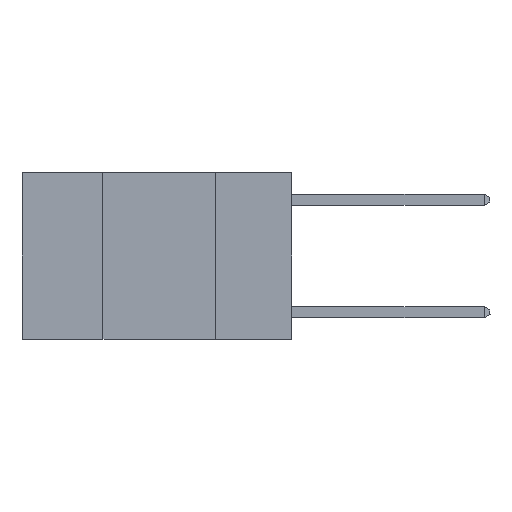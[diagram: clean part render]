
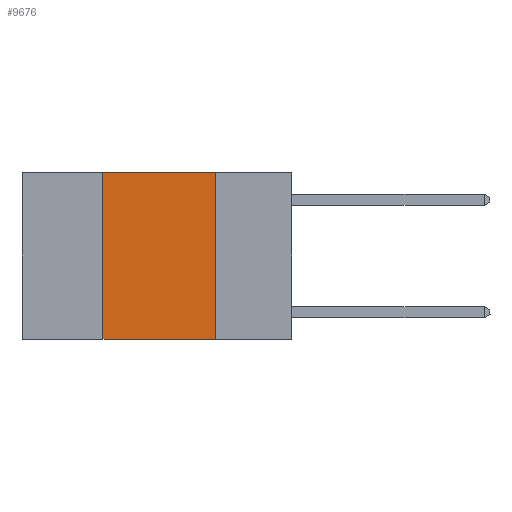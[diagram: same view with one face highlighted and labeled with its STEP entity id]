
A CAD part, left-side view. The second image highlights one B-rep face of the part: STEP entity #9676.
In plain terms, the highlighted planar face has unit normal (-1, 0, 0).
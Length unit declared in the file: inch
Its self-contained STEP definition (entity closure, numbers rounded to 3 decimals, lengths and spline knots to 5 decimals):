
#688 = DIRECTION ( 'NONE',  ( 0., 0., 1. ) ) ;
#775 = EDGE_CURVE ( 'NONE', #9578, #14769, #13753, .T. ) ;
#1675 = FACE_OUTER_BOUND ( 'NONE', #10880, .T. ) ;
#1906 = ORIENTED_EDGE ( 'NONE', *, *, #775, .F. ) ;
#2052 = CARTESIAN_POINT ( 'NONE',  ( 0., 0.17, -0.37 ) ) ;
#2343 = ORIENTED_EDGE ( 'NONE', *, *, #8108, .F. ) ;
#3382 = CARTESIAN_POINT ( 'NONE',  ( 0., 0.42, 0. ) ) ;
#4011 = DIRECTION ( 'NONE',  ( 0., 0., -1. ) ) ;
#4196 = DIRECTION ( 'NONE',  ( 0., 0., -1. ) ) ;
#4293 = VECTOR ( 'NONE', #688, 39.37008 ) ;
#4653 = VECTOR ( 'NONE', #15458, 39.37008 ) ;
#4660 = LINE ( 'NONE', #11481, #14763 ) ;
#4905 = CARTESIAN_POINT ( 'NONE',  ( 0., 0.6, -0.37 ) ) ;
#5914 = ORIENTED_EDGE ( 'NONE', *, *, #16284, .T. ) ;
#8107 = DIRECTION ( 'NONE',  ( 1., 0., 0. ) ) ;
#8108 = EDGE_CURVE ( 'NONE', #10949, #14846, #8243, .T. ) ;
#8243 = LINE ( 'NONE', #3382, #4293 ) ;
#8591 = LINE ( 'NONE', #4905, #4653 ) ;
#9578 = VERTEX_POINT ( 'NONE', #11880 ) ;
#9676 = ADVANCED_FACE ( 'NONE', ( #1675 ), #13347, .F. ) ;
#9982 = EDGE_CURVE ( 'NONE', #14846, #9578, #4660, .T. ) ;
#10280 = VECTOR ( 'NONE', #4196, 39.37008 ) ;
#10859 = AXIS2_PLACEMENT_3D ( 'NONE', #15958, #8107, #4011 ) ;
#10867 = CARTESIAN_POINT ( 'NONE',  ( 0., 0.42, -0.37 ) ) ;
#10880 = EDGE_LOOP ( 'NONE', ( #1906, #12571, #2343, #5914 ) ) ;
#10949 = VERTEX_POINT ( 'NONE', #10867 ) ;
#11481 = CARTESIAN_POINT ( 'NONE',  ( 0., 0.6, 0. ) ) ;
#11880 = CARTESIAN_POINT ( 'NONE',  ( 0., 0.17, 0. ) ) ;
#12571 = ORIENTED_EDGE ( 'NONE', *, *, #9982, .F. ) ;
#12799 = DIRECTION ( 'NONE',  ( 0., -1., 0. ) ) ;
#12908 = CARTESIAN_POINT ( 'NONE',  ( 0., 0.42, 0. ) ) ;
#13347 = PLANE ( 'NONE',  #10859 ) ;
#13753 = LINE ( 'NONE', #14409, #10280 ) ;
#14409 = CARTESIAN_POINT ( 'NONE',  ( 0., 0.17, 0. ) ) ;
#14763 = VECTOR ( 'NONE', #12799, 39.37008 ) ;
#14769 = VERTEX_POINT ( 'NONE', #2052 ) ;
#14846 = VERTEX_POINT ( 'NONE', #12908 ) ;
#15458 = DIRECTION ( 'NONE',  ( 0., -1., 0. ) ) ;
#15958 = CARTESIAN_POINT ( 'NONE',  ( 0., 0.6, 0. ) ) ;
#16284 = EDGE_CURVE ( 'NONE', #10949, #14769, #8591, .T. ) ;
